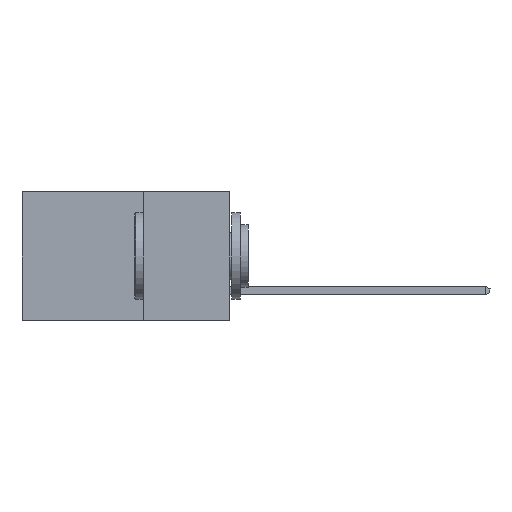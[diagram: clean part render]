
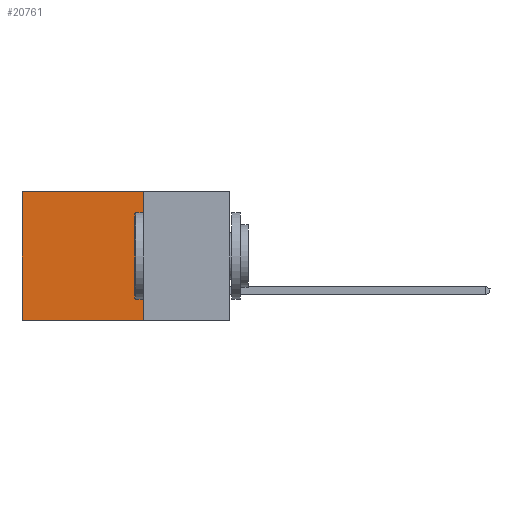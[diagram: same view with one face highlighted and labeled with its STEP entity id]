
A CAD part, left-side view. The second image highlights one B-rep face of the part: STEP entity #20761.
In plain terms, the highlighted planar face has unit normal (-1, 0, 0).
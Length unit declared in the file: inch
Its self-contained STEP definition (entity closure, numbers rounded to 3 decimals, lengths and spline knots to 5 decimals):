
#75 = DIRECTION ( 'NONE',  ( 0., 0., -1. ) ) ;
#130 = VERTEX_POINT ( 'NONE', #1017 ) ;
#1017 = CARTESIAN_POINT ( 'NONE',  ( 0.2615, 0.25, -0.37 ) ) ;
#1435 = ORIENTED_EDGE ( 'NONE', *, *, #4170, .F. ) ;
#1463 = CARTESIAN_POINT ( 'NONE',  ( 0.2615, 0.6, 0. ) ) ;
#2229 = DIRECTION ( 'NONE',  ( 0., 0., -1. ) ) ;
#2370 = ORIENTED_EDGE ( 'NONE', *, *, #18867, .T. ) ;
#2473 = DIRECTION ( 'NONE',  ( 0., 1., 0. ) ) ;
#3113 = VERTEX_POINT ( 'NONE', #14755 ) ;
#3638 = CARTESIAN_POINT ( 'NONE',  ( 0.2615, 0.25, 0. ) ) ;
#4094 = DIRECTION ( 'NONE',  ( 0., 1., 0. ) ) ;
#4170 = EDGE_CURVE ( 'NONE', #3113, #130, #16831, .T. ) ;
#6785 = FACE_OUTER_BOUND ( 'NONE', #19425, .T. ) ;
#7261 = CARTESIAN_POINT ( 'NONE',  ( 0.2615, 0.25, -0.37 ) ) ;
#7644 = ORIENTED_EDGE ( 'NONE', *, *, #17974, .T. ) ;
#7973 = CARTESIAN_POINT ( 'NONE',  ( 0.2615, 0.25, -0.37 ) ) ;
#9311 = ORIENTED_EDGE ( 'NONE', *, *, #18161, .F. ) ;
#9658 = VECTOR ( 'NONE', #2229, 39.37008 ) ;
#10155 = CARTESIAN_POINT ( 'NONE',  ( 0.2615, 0.6, -0.37 ) ) ;
#11594 = DIRECTION ( 'NONE',  ( 0., 0., -1. ) ) ;
#11708 = VERTEX_POINT ( 'NONE', #1463 ) ;
#11765 = CARTESIAN_POINT ( 'NONE',  ( 0.2615, 0.6, -0.37 ) ) ;
#12260 = VERTEX_POINT ( 'NONE', #10155 ) ;
#12898 = PLANE ( 'NONE',  #19982 ) ;
#13794 = VECTOR ( 'NONE', #2473, 39.37008 ) ;
#14755 = CARTESIAN_POINT ( 'NONE',  ( 0.2615, 0.25, 0. ) ) ;
#14929 = CARTESIAN_POINT ( 'NONE',  ( 0.2615, 0.25, -0.37 ) ) ;
#15809 = VECTOR ( 'NONE', #75, 39.37008 ) ;
#16196 = DIRECTION ( 'NONE',  ( 1., 0., 0. ) ) ;
#16831 = LINE ( 'NONE', #14929, #9658 ) ;
#17974 = EDGE_CURVE ( 'NONE', #11708, #12260, #19880, .T. ) ;
#18161 = EDGE_CURVE ( 'NONE', #130, #12260, #20212, .T. ) ;
#18692 = LINE ( 'NONE', #3638, #13794 ) ;
#18867 = EDGE_CURVE ( 'NONE', #3113, #11708, #18692, .T. ) ;
#18885 = VECTOR ( 'NONE', #4094, 39.37008 ) ;
#19425 = EDGE_LOOP ( 'NONE', ( #7644, #9311, #1435, #2370 ) ) ;
#19880 = LINE ( 'NONE', #11765, #15809 ) ;
#19982 = AXIS2_PLACEMENT_3D ( 'NONE', #7973, #16196, #11594 ) ;
#20212 = LINE ( 'NONE', #7261, #18885 ) ;
#20761 = ADVANCED_FACE ( 'NONE', ( #6785 ), #12898, .F. ) ;
